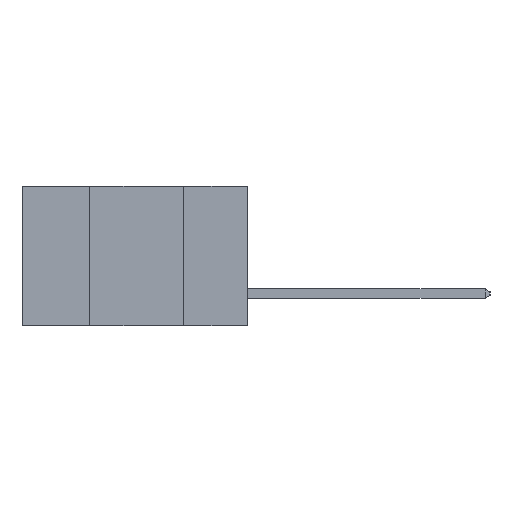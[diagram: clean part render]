
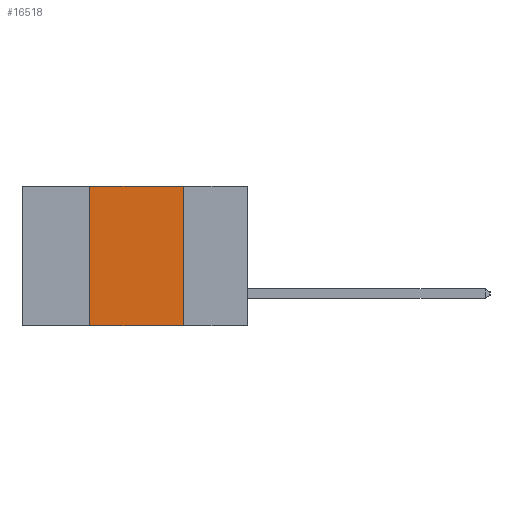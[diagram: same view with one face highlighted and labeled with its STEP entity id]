
A CAD part, left-side view. The second image highlights one B-rep face of the part: STEP entity #16518.
In plain terms, the highlighted planar face has unit normal (-1, 0, 0).
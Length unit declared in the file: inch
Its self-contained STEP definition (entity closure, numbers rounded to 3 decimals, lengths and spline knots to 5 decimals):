
#704 = DIRECTION ( 'NONE',  ( 0., -1., 0. ) ) ;
#881 = CARTESIAN_POINT ( 'NONE',  ( 0., 0.6, 0. ) ) ;
#989 = EDGE_CURVE ( 'NONE', #9973, #13936, #25572, .T. ) ;
#1500 = ORIENTED_EDGE ( 'NONE', *, *, #24751, .F. ) ;
#4150 = CARTESIAN_POINT ( 'NONE',  ( 0., 0.42, -0.37 ) ) ;
#4382 = CARTESIAN_POINT ( 'NONE',  ( 0., 0.17, 0. ) ) ;
#4505 = VECTOR ( 'NONE', #26781, 39.37008 ) ;
#5715 = ORIENTED_EDGE ( 'NONE', *, *, #989, .T. ) ;
#6054 = EDGE_CURVE ( 'NONE', #8418, #25515, #12071, .T. ) ;
#6665 = CARTESIAN_POINT ( 'NONE',  ( 0., 0.42, 0. ) ) ;
#7721 = EDGE_CURVE ( 'NONE', #25515, #13936, #19398, .T. ) ;
#8418 = VERTEX_POINT ( 'NONE', #27901 ) ;
#8439 = FACE_OUTER_BOUND ( 'NONE', #26704, .T. ) ;
#9276 = ORIENTED_EDGE ( 'NONE', *, *, #6054, .F. ) ;
#9313 = DIRECTION ( 'NONE',  ( 0., -1., 0. ) ) ;
#9973 = VERTEX_POINT ( 'NONE', #4150 ) ;
#12071 = LINE ( 'NONE', #881, #24617 ) ;
#13936 = VERTEX_POINT ( 'NONE', #16991 ) ;
#14896 = DIRECTION ( 'NONE',  ( 1., 0., 0. ) ) ;
#16518 = ADVANCED_FACE ( 'NONE', ( #8439 ), #29860, .F. ) ;
#16991 = CARTESIAN_POINT ( 'NONE',  ( 0., 0.17, -0.37 ) ) ;
#18900 = VECTOR ( 'NONE', #9313, 39.37008 ) ;
#19398 = LINE ( 'NONE', #21258, #25287 ) ;
#19509 = LINE ( 'NONE', #6665, #4505 ) ;
#20283 = ORIENTED_EDGE ( 'NONE', *, *, #7721, .F. ) ;
#20705 = DIRECTION ( 'NONE',  ( 0., 0., -1. ) ) ;
#21258 = CARTESIAN_POINT ( 'NONE',  ( 0., 0.17, 0. ) ) ;
#23033 = CARTESIAN_POINT ( 'NONE',  ( 0., 0.6, -0.37 ) ) ;
#24419 = AXIS2_PLACEMENT_3D ( 'NONE', #24842, #14896, #32340 ) ;
#24617 = VECTOR ( 'NONE', #704, 39.37008 ) ;
#24751 = EDGE_CURVE ( 'NONE', #9973, #8418, #19509, .T. ) ;
#24842 = CARTESIAN_POINT ( 'NONE',  ( 0., 0.6, 0. ) ) ;
#25287 = VECTOR ( 'NONE', #20705, 39.37008 ) ;
#25515 = VERTEX_POINT ( 'NONE', #4382 ) ;
#25572 = LINE ( 'NONE', #23033, #18900 ) ;
#26704 = EDGE_LOOP ( 'NONE', ( #20283, #9276, #1500, #5715 ) ) ;
#26781 = DIRECTION ( 'NONE',  ( 0., 0., 1. ) ) ;
#27901 = CARTESIAN_POINT ( 'NONE',  ( 0., 0.42, 0. ) ) ;
#29860 = PLANE ( 'NONE',  #24419 ) ;
#32340 = DIRECTION ( 'NONE',  ( 0., 0., -1. ) ) ;
